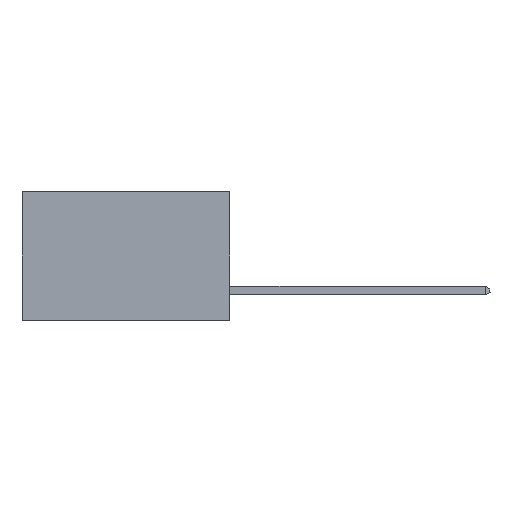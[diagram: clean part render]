
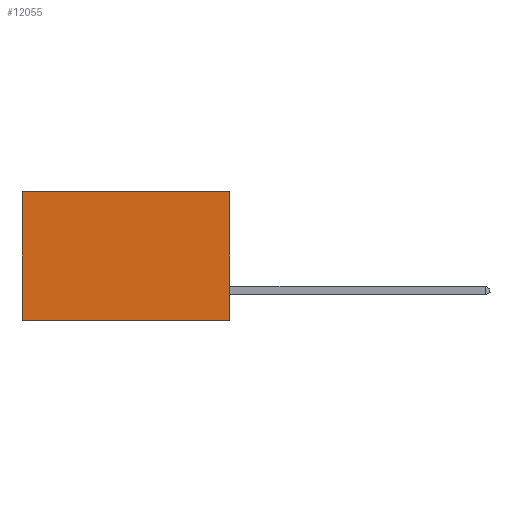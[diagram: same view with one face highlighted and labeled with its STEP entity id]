
A CAD part, left-side view. The second image highlights one B-rep face of the part: STEP entity #12055.
In plain terms, the highlighted planar face has unit normal (-1, 0, 0).
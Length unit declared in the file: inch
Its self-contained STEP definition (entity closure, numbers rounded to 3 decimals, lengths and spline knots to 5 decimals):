
#161 = ORIENTED_EDGE ( 'NONE', *, *, #9029, .F. ) ;
#1641 = VECTOR ( 'NONE', #1990, 39.37008 ) ;
#1990 = DIRECTION ( 'NONE',  ( 0., 1., 0. ) ) ;
#2473 = LINE ( 'NONE', #14425, #5584 ) ;
#2593 = DIRECTION ( 'NONE',  ( 0., 1., 0. ) ) ;
#2693 = DIRECTION ( 'NONE',  ( 0., 0., -1. ) ) ;
#2939 = CARTESIAN_POINT ( 'NONE',  ( 0.298, 0., -0.37 ) ) ;
#3225 = DIRECTION ( 'NONE',  ( 0., 0., -1. ) ) ;
#3824 = LINE ( 'NONE', #9764, #13650 ) ;
#5584 = VECTOR ( 'NONE', #2593, 39.37008 ) ;
#5765 = VERTEX_POINT ( 'NONE', #9867 ) ;
#5832 = ORIENTED_EDGE ( 'NONE', *, *, #16822, .T. ) ;
#7021 = FACE_OUTER_BOUND ( 'NONE', #10605, .T. ) ;
#7343 = EDGE_CURVE ( 'NONE', #16744, #15723, #2473, .T. ) ;
#8210 = ORIENTED_EDGE ( 'NONE', *, *, #8687, .T. ) ;
#8687 = EDGE_CURVE ( 'NONE', #10707, #15723, #3824, .T. ) ;
#9029 = EDGE_CURVE ( 'NONE', #5765, #16744, #17144, .T. ) ;
#9413 = PLANE ( 'NONE',  #14793 ) ;
#9764 = CARTESIAN_POINT ( 'NONE',  ( 0.298, 0.6, 0. ) ) ;
#9867 = CARTESIAN_POINT ( 'NONE',  ( 0.298, 0., 0. ) ) ;
#10605 = EDGE_LOOP ( 'NONE', ( #8210, #11935, #161, #5832 ) ) ;
#10611 = CARTESIAN_POINT ( 'NONE',  ( 0.298, 0., 0. ) ) ;
#10707 = VERTEX_POINT ( 'NONE', #13098 ) ;
#10792 = CARTESIAN_POINT ( 'NONE',  ( 0.298, 0., 0. ) ) ;
#11629 = LINE ( 'NONE', #16587, #1641 ) ;
#11935 = ORIENTED_EDGE ( 'NONE', *, *, #7343, .F. ) ;
#12055 = ADVANCED_FACE ( 'NONE', ( #7021 ), #9413, .F. ) ;
#12191 = DIRECTION ( 'NONE',  ( 1., 0., 0. ) ) ;
#12247 = DIRECTION ( 'NONE',  ( 0., 0., -1. ) ) ;
#13098 = CARTESIAN_POINT ( 'NONE',  ( 0.298, 0.6, 0. ) ) ;
#13650 = VECTOR ( 'NONE', #3225, 39.37008 ) ;
#14051 = VECTOR ( 'NONE', #2693, 39.37008 ) ;
#14425 = CARTESIAN_POINT ( 'NONE',  ( 0.298, 0., -0.37 ) ) ;
#14793 = AXIS2_PLACEMENT_3D ( 'NONE', #10792, #12191, #12247 ) ;
#14868 = CARTESIAN_POINT ( 'NONE',  ( 0.298, 0.6, -0.37 ) ) ;
#15723 = VERTEX_POINT ( 'NONE', #14868 ) ;
#16587 = CARTESIAN_POINT ( 'NONE',  ( 0.298, 0., 0. ) ) ;
#16744 = VERTEX_POINT ( 'NONE', #2939 ) ;
#16822 = EDGE_CURVE ( 'NONE', #5765, #10707, #11629, .T. ) ;
#17144 = LINE ( 'NONE', #10611, #14051 ) ;
